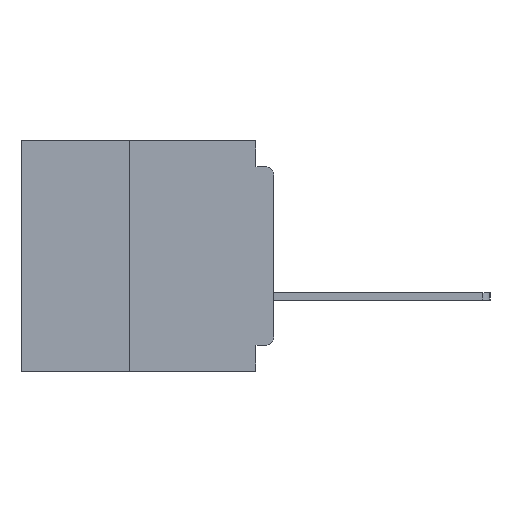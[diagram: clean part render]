
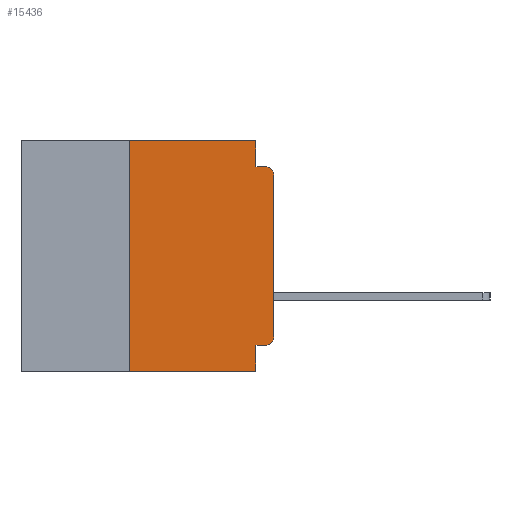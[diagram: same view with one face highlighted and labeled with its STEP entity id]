
A CAD part, left-side view. The second image highlights one B-rep face of the part: STEP entity #15436.
In plain terms, the highlighted planar face has unit normal (-1, 0, 0).
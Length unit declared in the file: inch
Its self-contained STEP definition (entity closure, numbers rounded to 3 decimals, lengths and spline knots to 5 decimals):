
#207 = VECTOR ( 'NONE', #24565, 39.37008 ) ;
#642 = LINE ( 'NONE', #24369, #35717 ) ;
#1482 = PLANE ( 'NONE',  #23292 ) ;
#3544 = CIRCLE ( 'NONE', #6202, 0.015 ) ;
#4213 = LINE ( 'NONE', #8690, #20055 ) ;
#4384 = DIRECTION ( 'NONE',  ( 1., 0., 0. ) ) ;
#4904 = VERTEX_POINT ( 'NONE', #8021 ) ;
#4961 = CARTESIAN_POINT ( 'NONE',  ( 0., 0.437, -0.4 ) ) ;
#5343 = ORIENTED_EDGE ( 'NONE', *, *, #8631, .T. ) ;
#5387 = EDGE_CURVE ( 'NONE', #13132, #22919, #26046, .T. ) ;
#5631 = CARTESIAN_POINT ( 'NONE',  ( 0., 0., -0.355 ) ) ;
#5826 = LINE ( 'NONE', #11139, #6726 ) ;
#6202 = AXIS2_PLACEMENT_3D ( 'NONE', #14484, #33917, #17322 ) ;
#6726 = VECTOR ( 'NONE', #30657, 39.37008 ) ;
#7017 = LINE ( 'NONE', #4961, #207 ) ;
#7398 = CARTESIAN_POINT ( 'NONE',  ( 0., 0., 0. ) ) ;
#7623 = DIRECTION ( 'NONE',  ( 0., 0., -1. ) ) ;
#8021 = CARTESIAN_POINT ( 'NONE',  ( 0., 0.015, -0.355 ) ) ;
#8075 = VECTOR ( 'NONE', #14059, 39.37008 ) ;
#8631 = EDGE_CURVE ( 'NONE', #18611, #22827, #35957, .T. ) ;
#8662 = VERTEX_POINT ( 'NONE', #20474 ) ;
#8690 = CARTESIAN_POINT ( 'NONE',  ( 0., 0.437, 0. ) ) ;
#8968 = LINE ( 'NONE', #27948, #8075 ) ;
#9252 = DIRECTION ( 'NONE',  ( -1., 0., 0. ) ) ;
#9442 = CARTESIAN_POINT ( 'NONE',  ( 0., 0.031, 0. ) ) ;
#9557 = EDGE_CURVE ( 'NONE', #4904, #18731, #29004, .T. ) ;
#9867 = ORIENTED_EDGE ( 'NONE', *, *, #33672, .T. ) ;
#10011 = AXIS2_PLACEMENT_3D ( 'NONE', #25968, #9252, #28733 ) ;
#11117 = DIRECTION ( 'NONE',  ( 0., 1., 0. ) ) ;
#11139 = CARTESIAN_POINT ( 'NONE',  ( 0., 0.25, -0.4 ) ) ;
#11491 = VECTOR ( 'NONE', #29706, 39.37008 ) ;
#12322 = ORIENTED_EDGE ( 'NONE', *, *, #31944, .F. ) ;
#13132 = VERTEX_POINT ( 'NONE', #35898 ) ;
#13616 = EDGE_CURVE ( 'NONE', #8662, #22208, #7017, .T. ) ;
#13952 = ORIENTED_EDGE ( 'NONE', *, *, #13616, .T. ) ;
#14059 = DIRECTION ( 'NONE',  ( 0., -1., 0. ) ) ;
#14180 = VECTOR ( 'NONE', #11117, 39.37008 ) ;
#14484 = CARTESIAN_POINT ( 'NONE',  ( 0., 0.015, -0.34 ) ) ;
#14534 = EDGE_CURVE ( 'NONE', #24464, #13132, #4213, .T. ) ;
#15347 = EDGE_LOOP ( 'NONE', ( #33880, #5343, #12322, #35056, #26191, #32176, #13952, #20158, #28494, #9867 ) ) ;
#15436 = ADVANCED_FACE ( 'NONE', ( #32139 ), #1482, .F. ) ;
#16392 = VERTEX_POINT ( 'NONE', #22883 ) ;
#16649 = CARTESIAN_POINT ( 'NONE',  ( 0., 0.031, -0.4 ) ) ;
#17322 = DIRECTION ( 'NONE',  ( 0., 0., -1. ) ) ;
#17713 = CARTESIAN_POINT ( 'NONE',  ( 0., 0., -0.06 ) ) ;
#18180 = CARTESIAN_POINT ( 'NONE',  ( 0., 0.031, -0.045 ) ) ;
#18611 = VERTEX_POINT ( 'NONE', #17713 ) ;
#18731 = VERTEX_POINT ( 'NONE', #23790 ) ;
#19526 = VECTOR ( 'NONE', #28924, 39.37008 ) ;
#20055 = VECTOR ( 'NONE', #28181, 39.37008 ) ;
#20158 = ORIENTED_EDGE ( 'NONE', *, *, #26744, .F. ) ;
#20474 = CARTESIAN_POINT ( 'NONE',  ( 0., 0.25, -0.4 ) ) ;
#20608 = CARTESIAN_POINT ( 'NONE',  ( 0., 0.015, -0.045 ) ) ;
#22208 = VERTEX_POINT ( 'NONE', #16649 ) ;
#22827 = VERTEX_POINT ( 'NONE', #20608 ) ;
#22883 = CARTESIAN_POINT ( 'NONE',  ( 0., 0., -0.34 ) ) ;
#22919 = VERTEX_POINT ( 'NONE', #18180 ) ;
#23077 = CARTESIAN_POINT ( 'NONE',  ( 0., 0.25, 0. ) ) ;
#23292 = AXIS2_PLACEMENT_3D ( 'NONE', #34993, #4384, #24020 ) ;
#23790 = CARTESIAN_POINT ( 'NONE',  ( 0., 0.031, -0.355 ) ) ;
#24020 = DIRECTION ( 'NONE',  ( 0., 0., -1. ) ) ;
#24369 = CARTESIAN_POINT ( 'NONE',  ( 0., 0.031, -0.4 ) ) ;
#24464 = VERTEX_POINT ( 'NONE', #23077 ) ;
#24565 = DIRECTION ( 'NONE',  ( 0., -1., 0. ) ) ;
#24719 = EDGE_CURVE ( 'NONE', #16392, #18611, #27191, .T. ) ;
#25968 = CARTESIAN_POINT ( 'NONE',  ( 0., 0.015, -0.06 ) ) ;
#26046 = LINE ( 'NONE', #9442, #19526 ) ;
#26191 = ORIENTED_EDGE ( 'NONE', *, *, #14534, .F. ) ;
#26744 = EDGE_CURVE ( 'NONE', #18731, #22208, #642, .T. ) ;
#27191 = LINE ( 'NONE', #7398, #11491 ) ;
#27948 = CARTESIAN_POINT ( 'NONE',  ( 0., 0., -0.045 ) ) ;
#28181 = DIRECTION ( 'NONE',  ( 0., -1., 0. ) ) ;
#28494 = ORIENTED_EDGE ( 'NONE', *, *, #9557, .F. ) ;
#28733 = DIRECTION ( 'NONE',  ( 0., 0., -1. ) ) ;
#28924 = DIRECTION ( 'NONE',  ( 0., 0., -1. ) ) ;
#29004 = LINE ( 'NONE', #5631, #14180 ) ;
#29706 = DIRECTION ( 'NONE',  ( 0., 0., 1. ) ) ;
#30657 = DIRECTION ( 'NONE',  ( 0., 0., 1. ) ) ;
#31944 = EDGE_CURVE ( 'NONE', #22919, #22827, #8968, .T. ) ;
#32139 = FACE_OUTER_BOUND ( 'NONE', #15347, .T. ) ;
#32176 = ORIENTED_EDGE ( 'NONE', *, *, #35958, .F. ) ;
#33672 = EDGE_CURVE ( 'NONE', #4904, #16392, #3544, .T. ) ;
#33880 = ORIENTED_EDGE ( 'NONE', *, *, #24719, .T. ) ;
#33917 = DIRECTION ( 'NONE',  ( -1., 0., 0. ) ) ;
#34993 = CARTESIAN_POINT ( 'NONE',  ( 0., 0.437, 0. ) ) ;
#35056 = ORIENTED_EDGE ( 'NONE', *, *, #5387, .F. ) ;
#35717 = VECTOR ( 'NONE', #7623, 39.37008 ) ;
#35898 = CARTESIAN_POINT ( 'NONE',  ( 0., 0.031, 0. ) ) ;
#35957 = CIRCLE ( 'NONE', #10011, 0.015 ) ;
#35958 = EDGE_CURVE ( 'NONE', #8662, #24464, #5826, .T. ) ;
